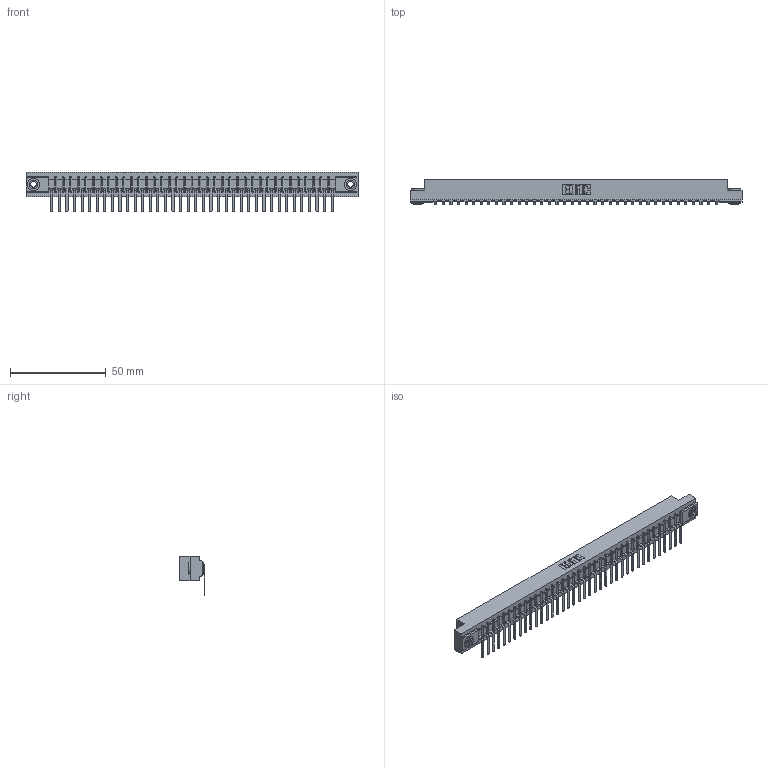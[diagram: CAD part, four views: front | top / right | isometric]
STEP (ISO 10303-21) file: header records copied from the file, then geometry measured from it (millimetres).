
FILE_DESCRIPTION (( 'STEP AP203' ), '1' );
FILE_NAME ('307-038-557-103.STEP', '2018-08-05T11:27:10', ( '' ), ( '' ), 'SwSTEP 2.0', 'SolidWorks 2016', '' );
FILE_SCHEMA (( 'CONFIG_CONTROL_DESIGN' ));
Length unit declared in the file: inch
Products named in the file (4): 307 Part_.156 Dia Mounting Holes; 307-290-002_557; 345-250-002_345-250-002-102; 307-038-557-103
Assembly tree (41 placements, depth 2):
  307-038-557-103
    307 Part_.156 Dia Mounting Holes
    307-290-002_557  x38
    345-250-002_345-250-002-102  x2
Bounding box: 173.58 x 13.36 x 20.66 mm (x, y, z)
Volume: 18649.7 mm3; surface area: 24277.4 mm2
Topology: 41 solids, 41 shells, 3173 faces, 9707 edges, 6362 vertices
Faces by surface type: plane 1880, cylinder 1207, sphere 78, cone 8
Entity records: 34989 total; most frequent: CARTESIAN_POINT 5881, ORIENTED_EDGE 5862, DIRECTION 5731, EDGE_CURVE 2931, LINE 2235, VECTOR 2235, VERTEX_POINT 1898, AXIS2_PLACEMENT_3D 1748
